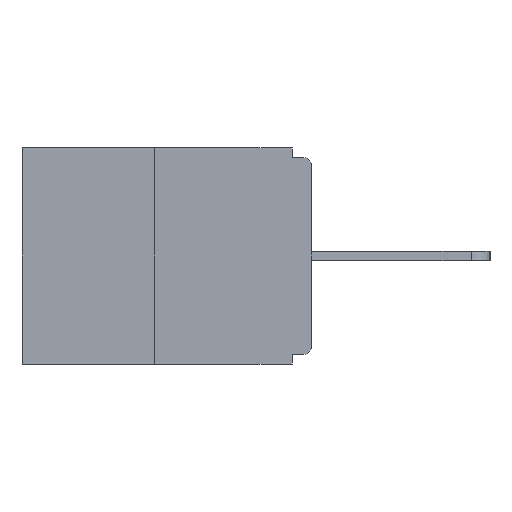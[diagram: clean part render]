
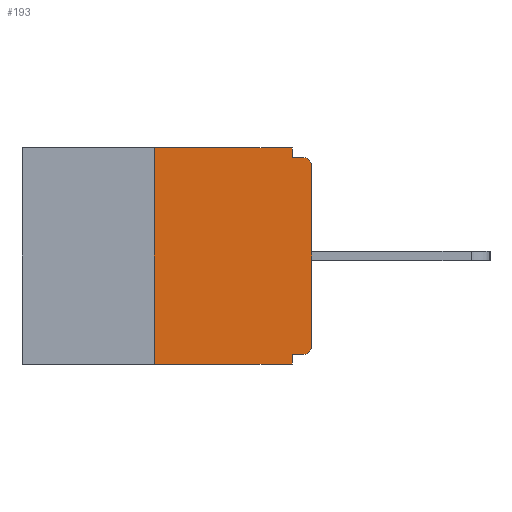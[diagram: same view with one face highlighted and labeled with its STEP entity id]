
A CAD part, left-side view. The second image highlights one B-rep face of the part: STEP entity #193.
In plain terms, the highlighted planar face has unit normal (-1, 0, 0).
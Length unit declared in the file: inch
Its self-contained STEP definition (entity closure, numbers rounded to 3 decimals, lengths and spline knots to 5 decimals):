
#193 = ADVANCED_FACE ( 'NONE', ( #11640 ), #12302, .F. ) ;
#446 = EDGE_CURVE ( 'NONE', #13518, #11821, #6561, .T. ) ;
#520 = CARTESIAN_POINT ( 'NONE',  ( 0., 0., -0.03 ) ) ;
#611 = VERTEX_POINT ( 'NONE', #6799 ) ;
#710 = VERTEX_POINT ( 'NONE', #11888 ) ;
#1082 = EDGE_LOOP ( 'NONE', ( #5735, #5760, #5798, #5823, #6076, #6223, #6552, #6621, #6946, #6969 ) ) ;
#1542 = CARTESIAN_POINT ( 'NONE',  ( 0., 0.031, -0.015 ) ) ;
#1821 = AXIS2_PLACEMENT_3D ( 'NONE', #6864, #6851, #12250 ) ;
#2136 = EDGE_CURVE ( 'NONE', #2960, #611, #6191, .T. ) ;
#2281 = LINE ( 'NONE', #10141, #8106 ) ;
#2423 = VERTEX_POINT ( 'NONE', #1542 ) ;
#2571 = VECTOR ( 'NONE', #5680, 39.37008 ) ;
#2960 = VERTEX_POINT ( 'NONE', #5147 ) ;
#3203 = DIRECTION ( 'NONE',  ( 0., 1., 0. ) ) ;
#3801 = CARTESIAN_POINT ( 'NONE',  ( 0., 0.015, -0.015 ) ) ;
#4033 = CARTESIAN_POINT ( 'NONE',  ( 0., 0.015, -0.313 ) ) ;
#4068 = AXIS2_PLACEMENT_3D ( 'NONE', #11831, #11447, #11122 ) ;
#4127 = EDGE_CURVE ( 'NONE', #6822, #13518, #10988, .T. ) ;
#4433 = VERTEX_POINT ( 'NONE', #9964 ) ;
#4521 = AXIS2_PLACEMENT_3D ( 'NONE', #4033, #11502, #5170 ) ;
#4606 = EDGE_CURVE ( 'NONE', #4433, #11821, #7011, .T. ) ;
#4802 = DIRECTION ( 'NONE',  ( 0., 0., -1. ) ) ;
#5090 = EDGE_CURVE ( 'NONE', #4433, #2960, #13133, .T. ) ;
#5147 = CARTESIAN_POINT ( 'NONE',  ( 0., 0.25, 0. ) ) ;
#5170 = DIRECTION ( 'NONE',  ( 0., 0., -1. ) ) ;
#5680 = DIRECTION ( 'NONE',  ( 0., 0., -1. ) ) ;
#5735 = ORIENTED_EDGE ( 'NONE', *, *, #2136, .F. ) ;
#5760 = ORIENTED_EDGE ( 'NONE', *, *, #5090, .F. ) ;
#5762 = EDGE_CURVE ( 'NONE', #6632, #13201, #6990, .T. ) ;
#5798 = ORIENTED_EDGE ( 'NONE', *, *, #4606, .T. ) ;
#5823 = ORIENTED_EDGE ( 'NONE', *, *, #446, .F. ) ;
#6076 = ORIENTED_EDGE ( 'NONE', *, *, #4127, .F. ) ;
#6100 = CARTESIAN_POINT ( 'NONE',  ( 0., 0.031, -0.343 ) ) ;
#6191 = LINE ( 'NONE', #7873, #9034 ) ;
#6223 = ORIENTED_EDGE ( 'NONE', *, *, #13998, .T. ) ;
#6474 = CARTESIAN_POINT ( 'NONE',  ( 0., 0.015, -0.328 ) ) ;
#6478 = CARTESIAN_POINT ( 'NONE',  ( 0., 0.031, -0.328 ) ) ;
#6552 = ORIENTED_EDGE ( 'NONE', *, *, #10789, .T. ) ;
#6561 = LINE ( 'NONE', #6100, #2571 ) ;
#6621 = ORIENTED_EDGE ( 'NONE', *, *, #5762, .T. ) ;
#6632 = VERTEX_POINT ( 'NONE', #520 ) ;
#6799 = CARTESIAN_POINT ( 'NONE',  ( 0., 0.031, 0. ) ) ;
#6822 = VERTEX_POINT ( 'NONE', #6474 ) ;
#6851 = DIRECTION ( 'NONE',  ( -1., 0., 0. ) ) ;
#6864 = CARTESIAN_POINT ( 'NONE',  ( 0., 0.015, -0.03 ) ) ;
#6868 = CARTESIAN_POINT ( 'NONE',  ( 0., 0., -0.328 ) ) ;
#6946 = ORIENTED_EDGE ( 'NONE', *, *, #7603, .F. ) ;
#6969 = ORIENTED_EDGE ( 'NONE', *, *, #13118, .F. ) ;
#6990 = CIRCLE ( 'NONE', #1821, 0.015 ) ;
#7011 = LINE ( 'NONE', #9152, #9513 ) ;
#7297 = DIRECTION ( 'NONE',  ( 0., -1., 0. ) ) ;
#7490 = CARTESIAN_POINT ( 'NONE',  ( 0., 0.031, -0.343 ) ) ;
#7603 = EDGE_CURVE ( 'NONE', #2423, #13201, #2281, .T. ) ;
#7671 = VECTOR ( 'NONE', #4802, 39.37008 ) ;
#7873 = CARTESIAN_POINT ( 'NONE',  ( 0., 0.46, 0. ) ) ;
#8000 = LINE ( 'NONE', #13154, #7671 ) ;
#8106 = VECTOR ( 'NONE', #11885, 39.37008 ) ;
#8177 = VECTOR ( 'NONE', #3203, 39.37008 ) ;
#9034 = VECTOR ( 'NONE', #7297, 39.37008 ) ;
#9065 = DIRECTION ( 'NONE',  ( 0., -1., 0. ) ) ;
#9152 = CARTESIAN_POINT ( 'NONE',  ( 0., 0.46, -0.343 ) ) ;
#9244 = VECTOR ( 'NONE', #10571, 39.37008 ) ;
#9513 = VECTOR ( 'NONE', #9065, 39.37008 ) ;
#9964 = CARTESIAN_POINT ( 'NONE',  ( 0., 0.25, -0.343 ) ) ;
#9976 = DIRECTION ( 'NONE',  ( 0., 0., 1. ) ) ;
#10141 = CARTESIAN_POINT ( 'NONE',  ( 0., 0., -0.015 ) ) ;
#10448 = VECTOR ( 'NONE', #9976, 39.37008 ) ;
#10571 = DIRECTION ( 'NONE',  ( 0., 0., 1. ) ) ;
#10573 = CARTESIAN_POINT ( 'NONE',  ( 0., 0., 0. ) ) ;
#10780 = CIRCLE ( 'NONE', #4521, 0.015 ) ;
#10789 = EDGE_CURVE ( 'NONE', #710, #6632, #11656, .T. ) ;
#10988 = LINE ( 'NONE', #6868, #8177 ) ;
#11122 = DIRECTION ( 'NONE',  ( 0., 0., -1. ) ) ;
#11296 = CARTESIAN_POINT ( 'NONE',  ( 0., 0.25, 0. ) ) ;
#11447 = DIRECTION ( 'NONE',  ( 1., 0., 0. ) ) ;
#11502 = DIRECTION ( 'NONE',  ( -1., 0., 0. ) ) ;
#11640 = FACE_OUTER_BOUND ( 'NONE', #1082, .T. ) ;
#11656 = LINE ( 'NONE', #10573, #9244 ) ;
#11821 = VERTEX_POINT ( 'NONE', #7490 ) ;
#11831 = CARTESIAN_POINT ( 'NONE',  ( 0., 0.46, 0. ) ) ;
#11885 = DIRECTION ( 'NONE',  ( 0., -1., 0. ) ) ;
#11888 = CARTESIAN_POINT ( 'NONE',  ( 0., 0., -0.313 ) ) ;
#12250 = DIRECTION ( 'NONE',  ( 0., 0., -1. ) ) ;
#12302 = PLANE ( 'NONE',  #4068 ) ;
#13118 = EDGE_CURVE ( 'NONE', #611, #2423, #8000, .T. ) ;
#13133 = LINE ( 'NONE', #11296, #10448 ) ;
#13154 = CARTESIAN_POINT ( 'NONE',  ( 0., 0.031, 0. ) ) ;
#13201 = VERTEX_POINT ( 'NONE', #3801 ) ;
#13518 = VERTEX_POINT ( 'NONE', #6478 ) ;
#13998 = EDGE_CURVE ( 'NONE', #6822, #710, #10780, .T. ) ;
